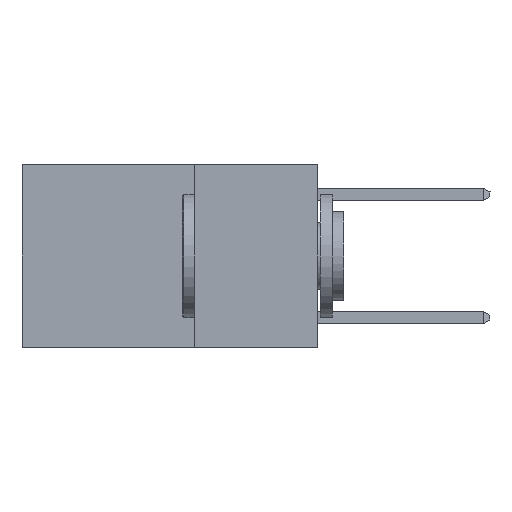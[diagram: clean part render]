
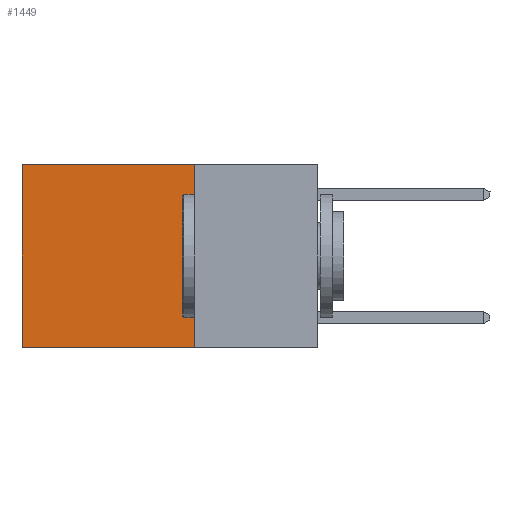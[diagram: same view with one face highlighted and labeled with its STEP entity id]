
A CAD part, left-side view. The second image highlights one B-rep face of the part: STEP entity #1449.
In plain terms, the highlighted planar face has unit normal (-1, 0, 0).
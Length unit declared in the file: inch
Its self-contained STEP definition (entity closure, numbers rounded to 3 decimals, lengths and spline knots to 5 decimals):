
#131 = VECTOR ( 'NONE', #7761, 39.37008 ) ;
#190 = LINE ( 'NONE', #1715, #131 ) ;
#240 = VERTEX_POINT ( 'NONE', #5265 ) ;
#332 = ORIENTED_EDGE ( 'NONE', *, *, #5722, .F. ) ;
#457 = EDGE_CURVE ( 'NONE', #8781, #240, #4006, .T. ) ;
#553 = ORIENTED_EDGE ( 'NONE', *, *, #457, .T. ) ;
#634 = PLANE ( 'NONE',  #5540 ) ;
#825 = CARTESIAN_POINT ( 'NONE',  ( 0.2625, 0.25, 0. ) ) ;
#834 = VERTEX_POINT ( 'NONE', #2157 ) ;
#905 = CARTESIAN_POINT ( 'NONE',  ( 0.2625, 0.25, 0. ) ) ;
#1087 = DIRECTION ( 'NONE',  ( 0., 1., 0. ) ) ;
#1277 = DIRECTION ( 'NONE',  ( 0., 0., -1. ) ) ;
#1449 = ADVANCED_FACE ( 'NONE', ( #4679 ), #634, .F. ) ;
#1715 = CARTESIAN_POINT ( 'NONE',  ( 0.2625, 0.25, -0.37 ) ) ;
#2157 = CARTESIAN_POINT ( 'NONE',  ( 0.2625, 0.25, -0.37 ) ) ;
#3452 = DIRECTION ( 'NONE',  ( 0., 0., -1. ) ) ;
#3721 = CARTESIAN_POINT ( 'NONE',  ( 0.2625, 0.25, 0. ) ) ;
#3816 = LINE ( 'NONE', #8313, #3932 ) ;
#3843 = CARTESIAN_POINT ( 'NONE',  ( 0.2625, 0.6, 0. ) ) ;
#3932 = VECTOR ( 'NONE', #4125, 39.37008 ) ;
#4006 = LINE ( 'NONE', #7939, #6750 ) ;
#4125 = DIRECTION ( 'NONE',  ( 0., 0., -1. ) ) ;
#4307 = EDGE_CURVE ( 'NONE', #6342, #834, #3816, .T. ) ;
#4433 = EDGE_LOOP ( 'NONE', ( #553, #332, #5760, #7991 ) ) ;
#4679 = FACE_OUTER_BOUND ( 'NONE', #4433, .T. ) ;
#5265 = CARTESIAN_POINT ( 'NONE',  ( 0.2625, 0.6, -0.37 ) ) ;
#5355 = DIRECTION ( 'NONE',  ( 1., 0., 0. ) ) ;
#5540 = AXIS2_PLACEMENT_3D ( 'NONE', #3721, #5355, #1277 ) ;
#5722 = EDGE_CURVE ( 'NONE', #834, #240, #190, .T. ) ;
#5760 = ORIENTED_EDGE ( 'NONE', *, *, #4307, .F. ) ;
#6342 = VERTEX_POINT ( 'NONE', #825 ) ;
#6750 = VECTOR ( 'NONE', #3452, 39.37008 ) ;
#6999 = EDGE_CURVE ( 'NONE', #6342, #8781, #7360, .T. ) ;
#7360 = LINE ( 'NONE', #905, #7462 ) ;
#7462 = VECTOR ( 'NONE', #1087, 39.37008 ) ;
#7761 = DIRECTION ( 'NONE',  ( 0., 1., 0. ) ) ;
#7939 = CARTESIAN_POINT ( 'NONE',  ( 0.2625, 0.6, 0. ) ) ;
#7991 = ORIENTED_EDGE ( 'NONE', *, *, #6999, .T. ) ;
#8313 = CARTESIAN_POINT ( 'NONE',  ( 0.2625, 0.25, 0. ) ) ;
#8781 = VERTEX_POINT ( 'NONE', #3843 ) ;
